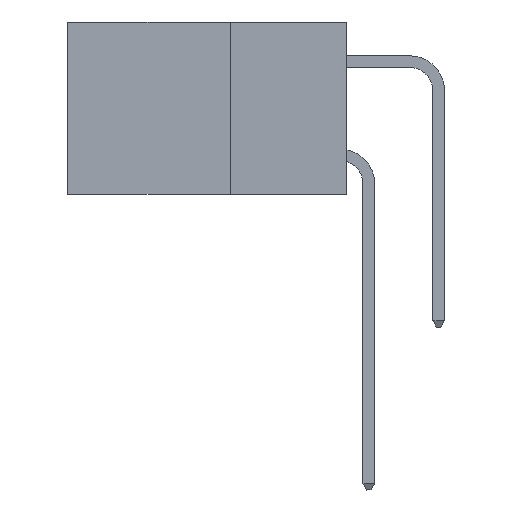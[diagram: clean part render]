
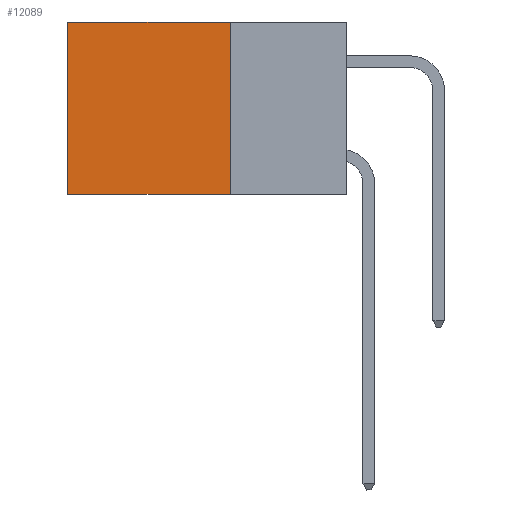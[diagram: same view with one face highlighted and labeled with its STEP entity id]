
A CAD part, left-side view. The second image highlights one B-rep face of the part: STEP entity #12089.
In plain terms, the highlighted planar face has unit normal (-1, 0, 0).
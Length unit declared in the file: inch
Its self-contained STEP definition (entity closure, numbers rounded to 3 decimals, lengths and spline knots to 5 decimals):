
#517 = CARTESIAN_POINT ( 'NONE',  ( 0.2875, 0.25, -0.37 ) ) ;
#723 = VECTOR ( 'NONE', #11560, 39.37008 ) ;
#942 = ORIENTED_EDGE ( 'NONE', *, *, #15737, .T. ) ;
#1350 = VERTEX_POINT ( 'NONE', #7194 ) ;
#2784 = VECTOR ( 'NONE', #6117, 39.37008 ) ;
#2966 = DIRECTION ( 'NONE',  ( 0., 0., -1. ) ) ;
#4359 = VERTEX_POINT ( 'NONE', #517 ) ;
#4609 = VERTEX_POINT ( 'NONE', #16686 ) ;
#4948 = CARTESIAN_POINT ( 'NONE',  ( 0.2875, 0.25, -0.37 ) ) ;
#5085 = ORIENTED_EDGE ( 'NONE', *, *, #27410, .F. ) ;
#5367 = EDGE_CURVE ( 'NONE', #4609, #1350, #13755, .T. ) ;
#6117 = DIRECTION ( 'NONE',  ( 0., 1., 0. ) ) ;
#6670 = LINE ( 'NONE', #4948, #723 ) ;
#7194 = CARTESIAN_POINT ( 'NONE',  ( 0.2875, 0.6, 0. ) ) ;
#7880 = FACE_OUTER_BOUND ( 'NONE', #24349, .T. ) ;
#10664 = EDGE_CURVE ( 'NONE', #4359, #27101, #6670, .T. ) ;
#11560 = DIRECTION ( 'NONE',  ( 0., 1., 0. ) ) ;
#12089 = ADVANCED_FACE ( 'NONE', ( #7880 ), #16334, .F. ) ;
#12431 = LINE ( 'NONE', #13884, #22471 ) ;
#13091 = CARTESIAN_POINT ( 'NONE',  ( 0.2875, 0.6, -0.37 ) ) ;
#13755 = LINE ( 'NONE', #19042, #2784 ) ;
#13884 = CARTESIAN_POINT ( 'NONE',  ( 0.2875, 0.6, 0. ) ) ;
#14152 = CARTESIAN_POINT ( 'NONE',  ( 0.2875, 0.25, 0. ) ) ;
#14432 = VECTOR ( 'NONE', #22699, 39.37008 ) ;
#14813 = AXIS2_PLACEMENT_3D ( 'NONE', #14152, #20497, #18464 ) ;
#15737 = EDGE_CURVE ( 'NONE', #1350, #27101, #12431, .T. ) ;
#16334 = PLANE ( 'NONE',  #14813 ) ;
#16686 = CARTESIAN_POINT ( 'NONE',  ( 0.2875, 0.25, 0. ) ) ;
#16819 = ORIENTED_EDGE ( 'NONE', *, *, #10664, .F. ) ;
#18464 = DIRECTION ( 'NONE',  ( 0., 0., -1. ) ) ;
#19042 = CARTESIAN_POINT ( 'NONE',  ( 0.2875, 0.25, 0. ) ) ;
#20497 = DIRECTION ( 'NONE',  ( 1., 0., 0. ) ) ;
#20543 = CARTESIAN_POINT ( 'NONE',  ( 0.2875, 0.25, 0. ) ) ;
#22471 = VECTOR ( 'NONE', #2966, 39.37008 ) ;
#22699 = DIRECTION ( 'NONE',  ( 0., 0., -1. ) ) ;
#22901 = ORIENTED_EDGE ( 'NONE', *, *, #5367, .T. ) ;
#24349 = EDGE_LOOP ( 'NONE', ( #942, #16819, #5085, #22901 ) ) ;
#25776 = LINE ( 'NONE', #20543, #14432 ) ;
#27101 = VERTEX_POINT ( 'NONE', #13091 ) ;
#27410 = EDGE_CURVE ( 'NONE', #4609, #4359, #25776, .T. ) ;
